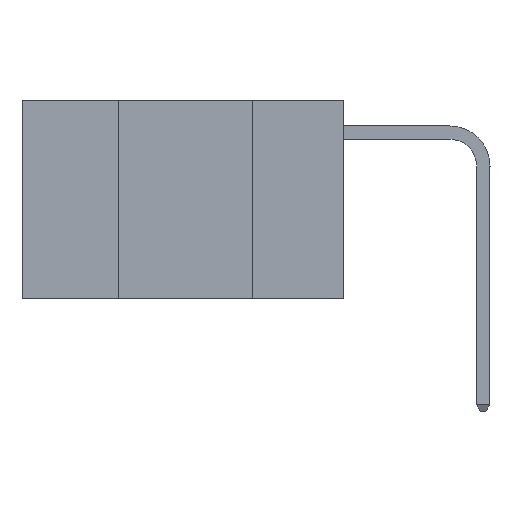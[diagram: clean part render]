
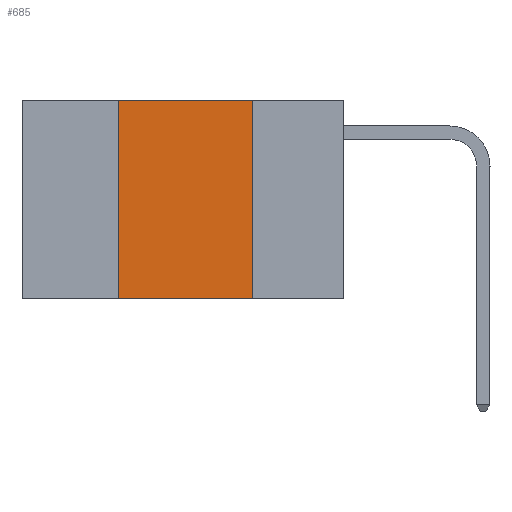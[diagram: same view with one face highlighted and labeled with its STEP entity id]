
A CAD part, left-side view. The second image highlights one B-rep face of the part: STEP entity #685.
In plain terms, the highlighted planar face has unit normal (-1, 0, 0).
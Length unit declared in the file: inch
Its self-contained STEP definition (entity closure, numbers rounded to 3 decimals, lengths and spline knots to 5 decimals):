
#442 = CARTESIAN_POINT ( 'NONE',  ( 0., 0.17, -0.37 ) ) ;
#493 = CARTESIAN_POINT ( 'NONE',  ( 0., 0.6, -0.37 ) ) ;
#685 = ADVANCED_FACE ( 'NONE', ( #3213 ), #7805, .F. ) ;
#1494 = DIRECTION ( 'NONE',  ( 0., 0., 1. ) ) ;
#2223 = VERTEX_POINT ( 'NONE', #6201 ) ;
#2464 = CARTESIAN_POINT ( 'NONE',  ( 0., 0.42, -0.37 ) ) ;
#2543 = AXIS2_PLACEMENT_3D ( 'NONE', #4893, #3652, #10629 ) ;
#2865 = LINE ( 'NONE', #8484, #14024 ) ;
#3213 = FACE_OUTER_BOUND ( 'NONE', #4016, .T. ) ;
#3584 = DIRECTION ( 'NONE',  ( 0., -1., 0. ) ) ;
#3652 = DIRECTION ( 'NONE',  ( 1., 0., 0. ) ) ;
#3890 = CARTESIAN_POINT ( 'NONE',  ( 0., 0.42, 0. ) ) ;
#3954 = EDGE_CURVE ( 'NONE', #13189, #2223, #8150, .T. ) ;
#4016 = EDGE_LOOP ( 'NONE', ( #4598, #4732, #4812, #4829 ) ) ;
#4598 = ORIENTED_EDGE ( 'NONE', *, *, #8416, .F. ) ;
#4732 = ORIENTED_EDGE ( 'NONE', *, *, #3954, .F. ) ;
#4812 = ORIENTED_EDGE ( 'NONE', *, *, #12826, .F. ) ;
#4829 = ORIENTED_EDGE ( 'NONE', *, *, #11409, .T. ) ;
#4893 = CARTESIAN_POINT ( 'NONE',  ( 0., 0.6, 0. ) ) ;
#5964 = VECTOR ( 'NONE', #3584, 39.37008 ) ;
#6201 = CARTESIAN_POINT ( 'NONE',  ( 0., 0.17, 0. ) ) ;
#6303 = DIRECTION ( 'NONE',  ( 0., -1., 0. ) ) ;
#6357 = DIRECTION ( 'NONE',  ( 0., 0., -1. ) ) ;
#7805 = PLANE ( 'NONE',  #2543 ) ;
#7908 = VERTEX_POINT ( 'NONE', #2464 ) ;
#8150 = LINE ( 'NONE', #10089, #5964 ) ;
#8242 = VERTEX_POINT ( 'NONE', #442 ) ;
#8416 = EDGE_CURVE ( 'NONE', #2223, #8242, #2865, .T. ) ;
#8484 = CARTESIAN_POINT ( 'NONE',  ( 0., 0.17, 0. ) ) ;
#9095 = VECTOR ( 'NONE', #1494, 39.37008 ) ;
#9455 = LINE ( 'NONE', #493, #9786 ) ;
#9786 = VECTOR ( 'NONE', #6303, 39.37008 ) ;
#10089 = CARTESIAN_POINT ( 'NONE',  ( 0., 0.6, 0. ) ) ;
#10629 = DIRECTION ( 'NONE',  ( 0., 0., -1. ) ) ;
#11409 = EDGE_CURVE ( 'NONE', #7908, #8242, #9455, .T. ) ;
#12305 = LINE ( 'NONE', #3890, #9095 ) ;
#12826 = EDGE_CURVE ( 'NONE', #7908, #13189, #12305, .T. ) ;
#13189 = VERTEX_POINT ( 'NONE', #13968 ) ;
#13968 = CARTESIAN_POINT ( 'NONE',  ( 0., 0.42, 0. ) ) ;
#14024 = VECTOR ( 'NONE', #6357, 39.37008 ) ;
